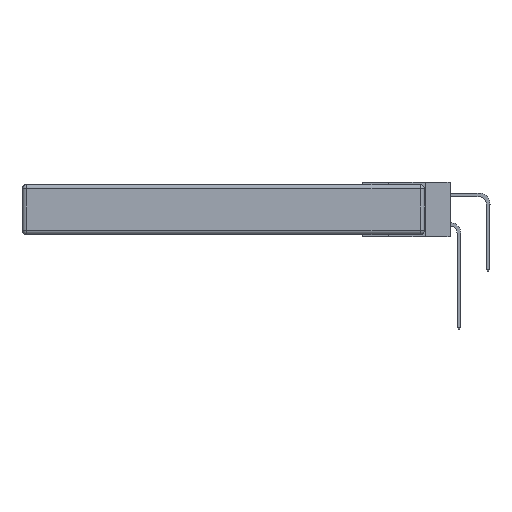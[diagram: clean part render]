
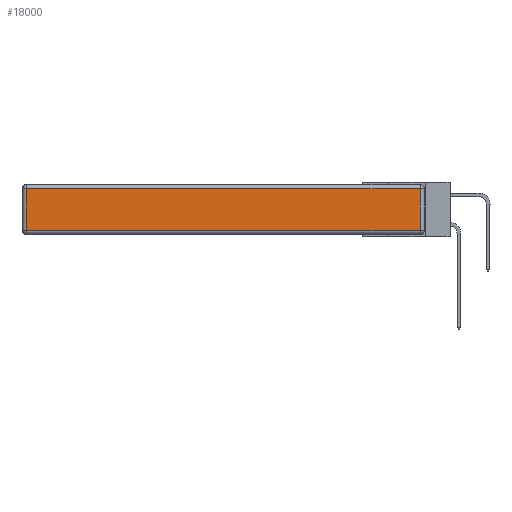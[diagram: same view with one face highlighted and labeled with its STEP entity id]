
A CAD part, left-side view. The second image highlights one B-rep face of the part: STEP entity #18000.
In plain terms, the highlighted planar face has unit normal (-1, 0, 0).
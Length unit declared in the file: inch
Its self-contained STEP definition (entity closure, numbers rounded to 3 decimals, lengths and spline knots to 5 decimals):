
#143 = VECTOR ( 'NONE', #21797, 39.37008 ) ;
#349 = VECTOR ( 'NONE', #13876, 39.37008 ) ;
#1494 = PLANE ( 'NONE',  #20462 ) ;
#1772 = EDGE_CURVE ( 'NONE', #25305, #12844, #22623, .T. ) ;
#2969 = CARTESIAN_POINT ( 'NONE',  ( 0., 0.03, -0.343 ) ) ;
#4951 = EDGE_CURVE ( 'NONE', #12844, #19010, #19623, .T. ) ;
#4952 = CARTESIAN_POINT ( 'NONE',  ( 0., 0.03, -0.03 ) ) ;
#7008 = EDGE_CURVE ( 'NONE', #14046, #25305, #23137, .T. ) ;
#7078 = CARTESIAN_POINT ( 'NONE',  ( 0., 2.72, -0.03 ) ) ;
#8671 = CARTESIAN_POINT ( 'NONE',  ( 0., 2.72, -0.313 ) ) ;
#9634 = DIRECTION ( 'NONE',  ( -1., 0., 0. ) ) ;
#11113 = ORIENTED_EDGE ( 'NONE', *, *, #1772, .T. ) ;
#11578 = VECTOR ( 'NONE', #22180, 39.37008 ) ;
#12009 = DIRECTION ( 'NONE',  ( 0., 0., 1. ) ) ;
#12844 = VERTEX_POINT ( 'NONE', #8671 ) ;
#13876 = DIRECTION ( 'NONE',  ( 0., 1., 0. ) ) ;
#14046 = VERTEX_POINT ( 'NONE', #4952 ) ;
#15028 = CARTESIAN_POINT ( 'NONE',  ( 0., 0., -0.313 ) ) ;
#15469 = LINE ( 'NONE', #2969, #143 ) ;
#15611 = FACE_OUTER_BOUND ( 'NONE', #17101, .T. ) ;
#16386 = VECTOR ( 'NONE', #25521, 39.37008 ) ;
#17101 = EDGE_LOOP ( 'NONE', ( #22441, #21496, #19770, #11113 ) ) ;
#18000 = ADVANCED_FACE ( 'NONE', ( #15611 ), #1494, .T. ) ;
#18105 = CARTESIAN_POINT ( 'NONE',  ( 0., 2.75, -0.03 ) ) ;
#19010 = VERTEX_POINT ( 'NONE', #21765 ) ;
#19623 = LINE ( 'NONE', #15028, #16386 ) ;
#19770 = ORIENTED_EDGE ( 'NONE', *, *, #7008, .T. ) ;
#20064 = CARTESIAN_POINT ( 'NONE',  ( 0., 2.72, -0.343 ) ) ;
#20462 = AXIS2_PLACEMENT_3D ( 'NONE', #22090, #9634, #12009 ) ;
#20734 = EDGE_CURVE ( 'NONE', #19010, #14046, #15469, .T. ) ;
#21496 = ORIENTED_EDGE ( 'NONE', *, *, #20734, .T. ) ;
#21765 = CARTESIAN_POINT ( 'NONE',  ( 0., 0.03, -0.313 ) ) ;
#21797 = DIRECTION ( 'NONE',  ( 0., 0., 1. ) ) ;
#22090 = CARTESIAN_POINT ( 'NONE',  ( 0., 0., -0.343 ) ) ;
#22180 = DIRECTION ( 'NONE',  ( 0., 0., -1. ) ) ;
#22441 = ORIENTED_EDGE ( 'NONE', *, *, #4951, .T. ) ;
#22623 = LINE ( 'NONE', #20064, #11578 ) ;
#23137 = LINE ( 'NONE', #18105, #349 ) ;
#25305 = VERTEX_POINT ( 'NONE', #7078 ) ;
#25521 = DIRECTION ( 'NONE',  ( 0., -1., 0. ) ) ;
